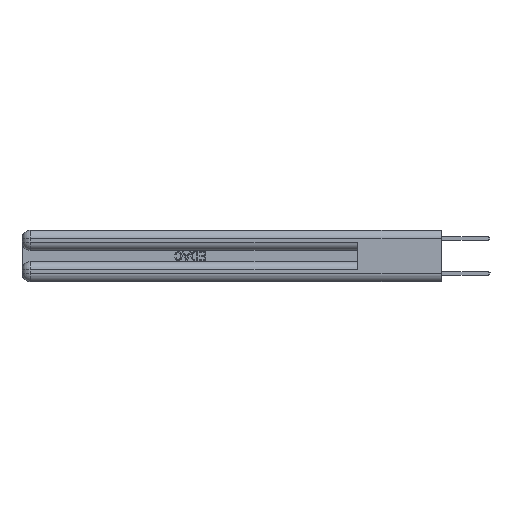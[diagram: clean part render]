
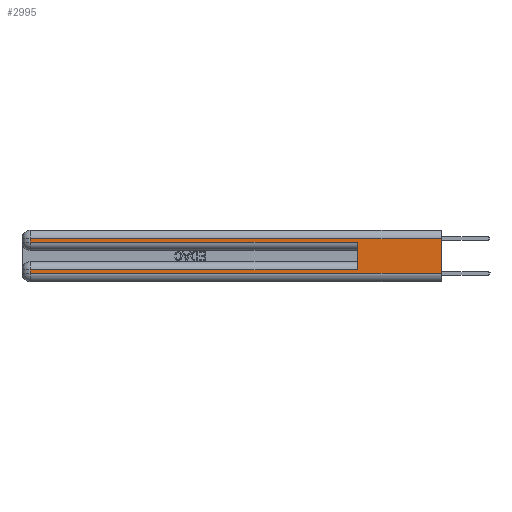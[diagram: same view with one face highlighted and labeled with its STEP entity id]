
A CAD part, left-side view. The second image highlights one B-rep face of the part: STEP entity #2995.
In plain terms, the highlighted planar face has unit normal (-1, 0, 0).
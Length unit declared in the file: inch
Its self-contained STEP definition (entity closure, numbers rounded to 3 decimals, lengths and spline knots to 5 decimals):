
#507 = LINE ( 'NONE', #26007, #16816 ) ;
#592 = ORIENTED_EDGE ( 'NONE', *, *, #31324, .F. ) ;
#717 = LINE ( 'NONE', #26855, #2279 ) ;
#1271 = CARTESIAN_POINT ( 'NONE',  ( 0., 2.94, 0.06 ) ) ;
#1435 = ORIENTED_EDGE ( 'NONE', *, *, #15425, .T. ) ;
#1626 = EDGE_LOOP ( 'NONE', ( #592, #25107, #12826, #1435, #23099, #26280, #13183, #11957 ) ) ;
#1670 = CARTESIAN_POINT ( 'NONE',  ( 0., 2.94, 0.31 ) ) ;
#1828 = LINE ( 'NONE', #15266, #25140 ) ;
#2215 = VECTOR ( 'NONE', #12140, 39.37008 ) ;
#2279 = VECTOR ( 'NONE', #31594, 39.37008 ) ;
#2995 = ADVANCED_FACE ( 'NONE', ( #25612 ), #5710, .F. ) ;
#3143 = CARTESIAN_POINT ( 'NONE',  ( 0., 0.6, 0.285 ) ) ;
#3749 = VERTEX_POINT ( 'NONE', #1670 ) ;
#4046 = VERTEX_POINT ( 'NONE', #6125 ) ;
#4146 = DIRECTION ( 'NONE',  ( 0., 0., -1. ) ) ;
#4504 = VERTEX_POINT ( 'NONE', #3143 ) ;
#5092 = CARTESIAN_POINT ( 'NONE',  ( 0., 0., 0.31 ) ) ;
#5307 = EDGE_CURVE ( 'NONE', #23668, #12619, #10656, .T. ) ;
#5710 = PLANE ( 'NONE',  #6503 ) ;
#6125 = CARTESIAN_POINT ( 'NONE',  ( 0., 2.94, 0.285 ) ) ;
#6345 = DIRECTION ( 'NONE',  ( 0., -1., 0. ) ) ;
#6444 = CARTESIAN_POINT ( 'NONE',  ( 0., 0., 0.37 ) ) ;
#6503 = AXIS2_PLACEMENT_3D ( 'NONE', #23083, #8187, #25608 ) ;
#7045 = CARTESIAN_POINT ( 'NONE',  ( 0., 0., 0.06 ) ) ;
#8187 = DIRECTION ( 'NONE',  ( 1., 0., 0. ) ) ;
#10656 = LINE ( 'NONE', #20817, #23124 ) ;
#11957 = ORIENTED_EDGE ( 'NONE', *, *, #22229, .T. ) ;
#12140 = DIRECTION ( 'NONE',  ( 0., -1., 0. ) ) ;
#12619 = VERTEX_POINT ( 'NONE', #13048 ) ;
#12826 = ORIENTED_EDGE ( 'NONE', *, *, #18711, .T. ) ;
#13048 = CARTESIAN_POINT ( 'NONE',  ( 0., 2.94, 0.085 ) ) ;
#13183 = ORIENTED_EDGE ( 'NONE', *, *, #30001, .T. ) ;
#15266 = CARTESIAN_POINT ( 'NONE',  ( 0., 2.94, 0.37 ) ) ;
#15425 = EDGE_CURVE ( 'NONE', #4046, #4504, #29413, .T. ) ;
#15869 = CARTESIAN_POINT ( 'NONE',  ( 0., 0., 0.06 ) ) ;
#16816 = VECTOR ( 'NONE', #18948, 39.37008 ) ;
#17468 = DIRECTION ( 'NONE',  ( 0., 0., -1. ) ) ;
#18711 = EDGE_CURVE ( 'NONE', #3749, #4046, #1828, .T. ) ;
#18948 = DIRECTION ( 'NONE',  ( 0., 0., -1. ) ) ;
#20817 = CARTESIAN_POINT ( 'NONE',  ( 0., 0., 0.085 ) ) ;
#20997 = VERTEX_POINT ( 'NONE', #7045 ) ;
#21519 = VECTOR ( 'NONE', #23750, 39.37008 ) ;
#21526 = VERTEX_POINT ( 'NONE', #1271 ) ;
#22229 = EDGE_CURVE ( 'NONE', #21526, #20997, #25363, .T. ) ;
#23069 = LINE ( 'NONE', #28396, #21519 ) ;
#23083 = CARTESIAN_POINT ( 'NONE',  ( 0., 0., 0.37 ) ) ;
#23099 = ORIENTED_EDGE ( 'NONE', *, *, #25894, .F. ) ;
#23124 = VECTOR ( 'NONE', #23657, 39.37008 ) ;
#23657 = DIRECTION ( 'NONE',  ( 0., 1., 0. ) ) ;
#23668 = VERTEX_POINT ( 'NONE', #31077 ) ;
#23750 = DIRECTION ( 'NONE',  ( 0., 1., 0. ) ) ;
#23812 = VECTOR ( 'NONE', #6345, 39.37008 ) ;
#24774 = CARTESIAN_POINT ( 'NONE',  ( 0., 0., 0.285 ) ) ;
#25107 = ORIENTED_EDGE ( 'NONE', *, *, #29516, .T. ) ;
#25140 = VECTOR ( 'NONE', #17468, 39.37008 ) ;
#25363 = LINE ( 'NONE', #15869, #23812 ) ;
#25608 = DIRECTION ( 'NONE',  ( 0., 0., -1. ) ) ;
#25612 = FACE_OUTER_BOUND ( 'NONE', #1626, .T. ) ;
#25718 = VECTOR ( 'NONE', #4146, 39.37008 ) ;
#25894 = EDGE_CURVE ( 'NONE', #23668, #4504, #717, .T. ) ;
#26007 = CARTESIAN_POINT ( 'NONE',  ( 0., 2.94, 0.37 ) ) ;
#26079 = LINE ( 'NONE', #6444, #25718 ) ;
#26138 = VERTEX_POINT ( 'NONE', #5092 ) ;
#26280 = ORIENTED_EDGE ( 'NONE', *, *, #5307, .T. ) ;
#26855 = CARTESIAN_POINT ( 'NONE',  ( 0., 0.6, 0.145 ) ) ;
#28396 = CARTESIAN_POINT ( 'NONE',  ( 0., 0., 0.31 ) ) ;
#29413 = LINE ( 'NONE', #24774, #2215 ) ;
#29516 = EDGE_CURVE ( 'NONE', #26138, #3749, #23069, .T. ) ;
#30001 = EDGE_CURVE ( 'NONE', #12619, #21526, #507, .T. ) ;
#31077 = CARTESIAN_POINT ( 'NONE',  ( 0., 0.6, 0.085 ) ) ;
#31324 = EDGE_CURVE ( 'NONE', #26138, #20997, #26079, .T. ) ;
#31594 = DIRECTION ( 'NONE',  ( 0., 0., 1. ) ) ;
